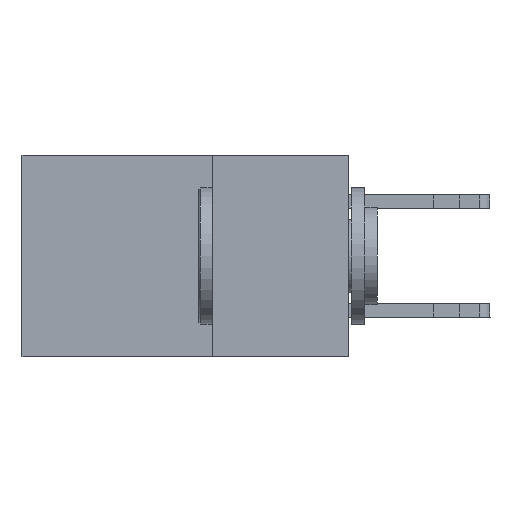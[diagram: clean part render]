
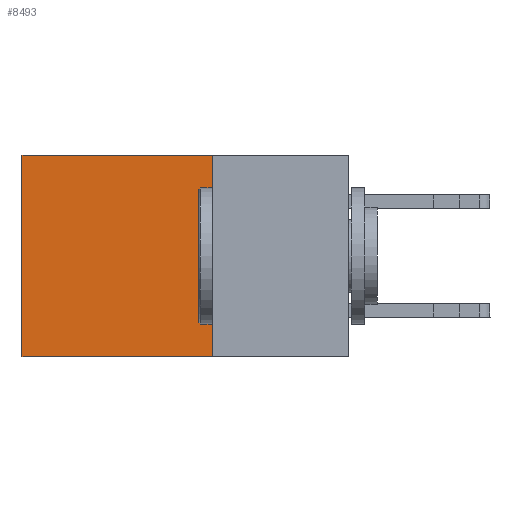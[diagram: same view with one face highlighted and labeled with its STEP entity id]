
A CAD part, left-side view. The second image highlights one B-rep face of the part: STEP entity #8493.
In plain terms, the highlighted planar face has unit normal (-1, 0, 0).
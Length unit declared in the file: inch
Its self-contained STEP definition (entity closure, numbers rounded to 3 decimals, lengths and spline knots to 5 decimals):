
#5 = CARTESIAN_POINT ( 'NONE',  ( 0.298, 0.25, 0. ) ) ;
#18 = CARTESIAN_POINT ( 'NONE',  ( 0.298, 0.25, 0. ) ) ;
#405 = VERTEX_POINT ( 'NONE', #17191 ) ;
#900 = ORIENTED_EDGE ( 'NONE', *, *, #11156, .F. ) ;
#1738 = LINE ( 'NONE', #5, #21579 ) ;
#2865 = DIRECTION ( 'NONE',  ( 0., 0., -1. ) ) ;
#3261 = VECTOR ( 'NONE', #18917, 39.37008 ) ;
#4178 = VERTEX_POINT ( 'NONE', #12958 ) ;
#5600 = EDGE_CURVE ( 'NONE', #20622, #405, #18619, .T. ) ;
#6003 = ORIENTED_EDGE ( 'NONE', *, *, #17490, .T. ) ;
#8493 = ADVANCED_FACE ( 'NONE', ( #11324 ), #19083, .F. ) ;
#9056 = CARTESIAN_POINT ( 'NONE',  ( 0.298, 0.25, -0.37 ) ) ;
#9146 = VECTOR ( 'NONE', #2865, 39.37008 ) ;
#9583 = CARTESIAN_POINT ( 'NONE',  ( 0.298, 0.6, 0. ) ) ;
#11156 = EDGE_CURVE ( 'NONE', #4178, #20622, #15775, .T. ) ;
#11324 = FACE_OUTER_BOUND ( 'NONE', #18491, .T. ) ;
#11496 = EDGE_CURVE ( 'NONE', #4178, #19796, #1738, .T. ) ;
#11726 = VECTOR ( 'NONE', #12758, 39.37008 ) ;
#12287 = DIRECTION ( 'NONE',  ( 0., 1., 0. ) ) ;
#12758 = DIRECTION ( 'NONE',  ( 0., 1., 0. ) ) ;
#12958 = CARTESIAN_POINT ( 'NONE',  ( 0.298, 0.25, 0. ) ) ;
#13712 = CARTESIAN_POINT ( 'NONE',  ( 0.298, 0.25, -0.37 ) ) ;
#13837 = DIRECTION ( 'NONE',  ( 1., 0., 0. ) ) ;
#15775 = LINE ( 'NONE', #17082, #9146 ) ;
#17082 = CARTESIAN_POINT ( 'NONE',  ( 0.298, 0.25, 0. ) ) ;
#17191 = CARTESIAN_POINT ( 'NONE',  ( 0.298, 0.6, -0.37 ) ) ;
#17324 = ORIENTED_EDGE ( 'NONE', *, *, #11496, .T. ) ;
#17454 = CARTESIAN_POINT ( 'NONE',  ( 0.298, 0.6, 0. ) ) ;
#17490 = EDGE_CURVE ( 'NONE', #19796, #405, #19562, .T. ) ;
#18491 = EDGE_LOOP ( 'NONE', ( #6003, #22703, #900, #17324 ) ) ;
#18619 = LINE ( 'NONE', #9056, #11726 ) ;
#18917 = DIRECTION ( 'NONE',  ( 0., 0., -1. ) ) ;
#19083 = PLANE ( 'NONE',  #19984 ) ;
#19562 = LINE ( 'NONE', #17454, #3261 ) ;
#19796 = VERTEX_POINT ( 'NONE', #9583 ) ;
#19984 = AXIS2_PLACEMENT_3D ( 'NONE', #18, #13837, #22760 ) ;
#20622 = VERTEX_POINT ( 'NONE', #13712 ) ;
#21579 = VECTOR ( 'NONE', #12287, 39.37008 ) ;
#22703 = ORIENTED_EDGE ( 'NONE', *, *, #5600, .F. ) ;
#22760 = DIRECTION ( 'NONE',  ( 0., 0., -1. ) ) ;
